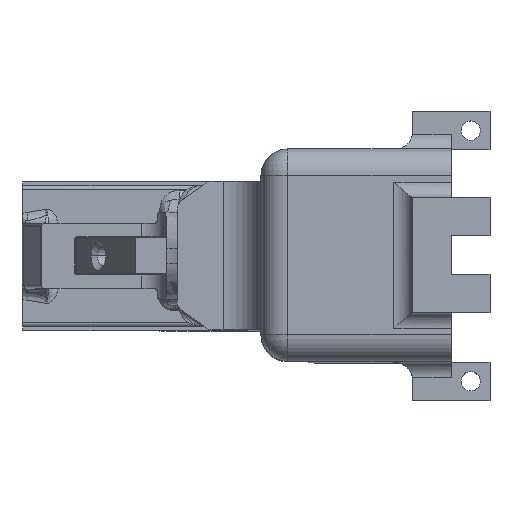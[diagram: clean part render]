
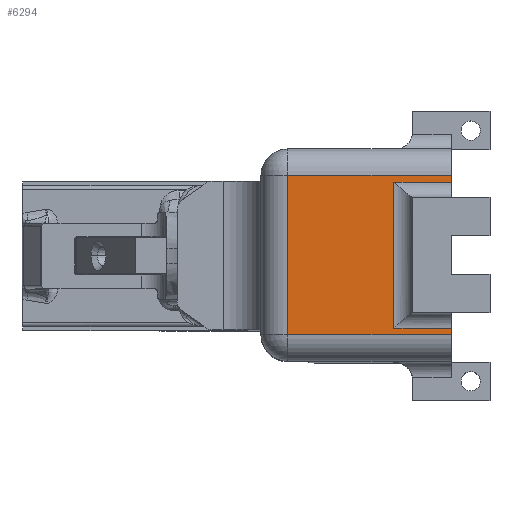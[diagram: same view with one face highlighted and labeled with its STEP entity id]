
A CAD part, top view. The second image highlights one B-rep face of the part: STEP entity #6294.
In plain terms, the highlighted planar face has unit normal (0, 0, 1).
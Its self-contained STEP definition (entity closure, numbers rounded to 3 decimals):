
#241 = ORIENTED_EDGE ( 'NONE', *, *, #12892, .T. ) ;
#513 = VECTOR ( 'NONE', #10686, 1000. ) ;
#526 = ORIENTED_EDGE ( 'NONE', *, *, #7362, .T. ) ;
#688 = CARTESIAN_POINT ( 'NONE',  ( 101.362, -20.148, 147.352 ) ) ;
#727 = VECTOR ( 'NONE', #2937, 1000. ) ;
#798 = VECTOR ( 'NONE', #6088, 1000. ) ;
#1555 = DIRECTION ( 'NONE',  ( -1., 0., 0. ) ) ;
#1614 = VECTOR ( 'NONE', #14887, 1000. ) ;
#1724 = CARTESIAN_POINT ( 'NONE',  ( 116.522, -60.353, 147.352 ) ) ;
#2037 = CARTESIAN_POINT ( 'NONE',  ( 116.522, -20.148, 147.352 ) ) ;
#2259 = DIRECTION ( 'NONE',  ( 0., 0., -1. ) ) ;
#2571 = VERTEX_POINT ( 'NONE', #9366 ) ;
#2937 = DIRECTION ( 'NONE',  ( 1., 0., 0. ) ) ;
#3567 = CARTESIAN_POINT ( 'NONE',  ( 101.362, -58.628, 147.352 ) ) ;
#3984 = EDGE_CURVE ( 'NONE', #9633, #13774, #4321, .T. ) ;
#4130 = CARTESIAN_POINT ( 'NONE',  ( 116.522, -18.424, 147.352 ) ) ;
#4321 = LINE ( 'NONE', #15318, #13390 ) ;
#4377 = VECTOR ( 'NONE', #14145, 1000. ) ;
#4476 = LINE ( 'NONE', #8547, #798 ) ;
#4928 = CARTESIAN_POINT ( 'NONE',  ( 106.362, -58.628, 147.352 ) ) ;
#5693 = ORIENTED_EDGE ( 'NONE', *, *, #10358, .T. ) ;
#5819 = CARTESIAN_POINT ( 'NONE',  ( 116.522, -11.424, 147.352 ) ) ;
#5838 = EDGE_CURVE ( 'NONE', #2571, #9008, #9669, .T. ) ;
#5915 = VERTEX_POINT ( 'NONE', #4130 ) ;
#6088 = DIRECTION ( 'NONE',  ( 0., 1., 0. ) ) ;
#6159 = LINE ( 'NONE', #5819, #12513 ) ;
#6294 = ADVANCED_FACE ( 'NONE', ( #11212 ), #8500, .F. ) ;
#7362 = EDGE_CURVE ( 'NONE', #13774, #11823, #15043, .T. ) ;
#7789 = LINE ( 'NONE', #8715, #1614 ) ;
#8068 = CARTESIAN_POINT ( 'NONE',  ( 0., -20.148, 147.352 ) ) ;
#8192 = CARTESIAN_POINT ( 'NONE',  ( 73.323, -60.353, 147.352 ) ) ;
#8500 = PLANE ( 'NONE',  #11731 ) ;
#8547 = CARTESIAN_POINT ( 'NONE',  ( 116.522, -11.424, 147.352 ) ) ;
#8715 = CARTESIAN_POINT ( 'NONE',  ( 73.323, -18.424, 147.352 ) ) ;
#8789 = ORIENTED_EDGE ( 'NONE', *, *, #5838, .T. ) ;
#8901 = EDGE_CURVE ( 'NONE', #9008, #10257, #11506, .T. ) ;
#9008 = VERTEX_POINT ( 'NONE', #3567 ) ;
#9366 = CARTESIAN_POINT ( 'NONE',  ( 116.522, -58.628, 147.352 ) ) ;
#9547 = DIRECTION ( 'NONE',  ( 0., 1., 0. ) ) ;
#9633 = VERTEX_POINT ( 'NONE', #12980 ) ;
#9669 = LINE ( 'NONE', #4928, #11790 ) ;
#10257 = VERTEX_POINT ( 'NONE', #12639 ) ;
#10358 = EDGE_CURVE ( 'NONE', #5915, #9633, #7789, .T. ) ;
#10368 = CARTESIAN_POINT ( 'NONE',  ( 116.522, -60.353, 147.352 ) ) ;
#10686 = DIRECTION ( 'NONE',  ( 1., 0., 0. ) ) ;
#10857 = DIRECTION ( 'NONE',  ( -1., 0., 0. ) ) ;
#11212 = FACE_OUTER_BOUND ( 'NONE', #12651, .T. ) ;
#11506 = LINE ( 'NONE', #688, #4377 ) ;
#11731 = AXIS2_PLACEMENT_3D ( 'NONE', #12140, #2259, #10857 ) ;
#11790 = VECTOR ( 'NONE', #1555, 1000. ) ;
#11823 = VERTEX_POINT ( 'NONE', #1724 ) ;
#12140 = CARTESIAN_POINT ( 'NONE',  ( 0., 0., 147.352 ) ) ;
#12513 = VECTOR ( 'NONE', #9547, 1000. ) ;
#12539 = ORIENTED_EDGE ( 'NONE', *, *, #8901, .T. ) ;
#12639 = CARTESIAN_POINT ( 'NONE',  ( 101.362, -20.148, 147.352 ) ) ;
#12651 = EDGE_LOOP ( 'NONE', ( #8789, #12539, #15854, #12963, #5693, #15279, #526, #241 ) ) ;
#12883 = LINE ( 'NONE', #8068, #513 ) ;
#12892 = EDGE_CURVE ( 'NONE', #11823, #2571, #4476, .T. ) ;
#12963 = ORIENTED_EDGE ( 'NONE', *, *, #14353, .T. ) ;
#12980 = CARTESIAN_POINT ( 'NONE',  ( 73.323, -18.424, 147.352 ) ) ;
#12987 = DIRECTION ( 'NONE',  ( 0., -1., 0. ) ) ;
#13390 = VECTOR ( 'NONE', #12987, 1000. ) ;
#13774 = VERTEX_POINT ( 'NONE', #8192 ) ;
#14145 = DIRECTION ( 'NONE',  ( 0., 1., 0. ) ) ;
#14353 = EDGE_CURVE ( 'NONE', #15685, #5915, #6159, .T. ) ;
#14887 = DIRECTION ( 'NONE',  ( -1., 0., 0. ) ) ;
#15043 = LINE ( 'NONE', #10368, #727 ) ;
#15279 = ORIENTED_EDGE ( 'NONE', *, *, #3984, .T. ) ;
#15318 = CARTESIAN_POINT ( 'NONE',  ( 73.323, 0., 147.352 ) ) ;
#15650 = EDGE_CURVE ( 'NONE', #10257, #15685, #12883, .T. ) ;
#15685 = VERTEX_POINT ( 'NONE', #2037 ) ;
#15854 = ORIENTED_EDGE ( 'NONE', *, *, #15650, .T. ) ;
